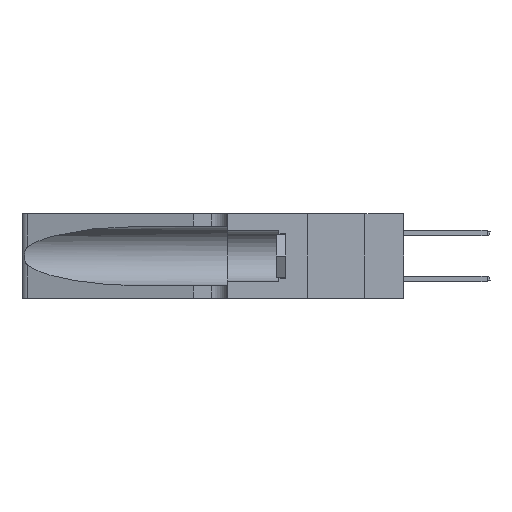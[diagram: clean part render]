
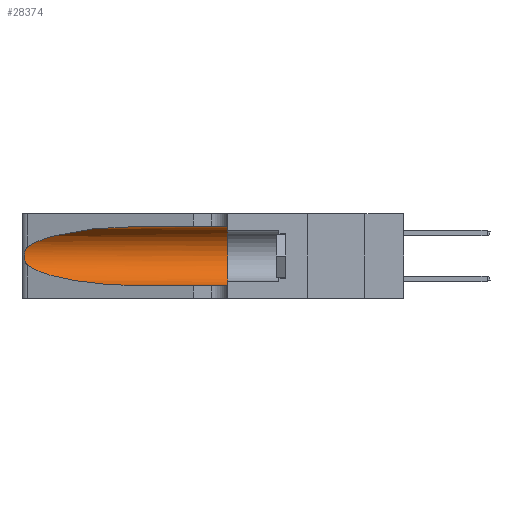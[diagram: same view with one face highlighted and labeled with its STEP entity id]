
A CAD part, left-side view. The second image highlights one B-rep face of the part: STEP entity #28374.
In plain terms, the highlighted cylindrical face has radius 3.308 mm (diameter 6.617 mm), a partial arc.
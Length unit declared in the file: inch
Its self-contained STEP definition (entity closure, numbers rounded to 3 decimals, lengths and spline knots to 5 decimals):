
#42 =( BOUNDED_CURVE ( )  B_SPLINE_CURVE ( 3, ( #224, #16903, #26453, #12285 ),
 .UNSPECIFIED., .F., .T. ) 
 B_SPLINE_CURVE_WITH_KNOTS ( ( 4, 4 ),
 ( 1.5708, 2.84003 ),
 .UNSPECIFIED. ) 
 CURVE ( )  GEOMETRIC_REPRESENTATION_ITEM ( )  RATIONAL_B_SPLINE_CURVE ( ( 1., 0.87, 0.87, 1. ) ) 
 REPRESENTATION_ITEM ( '' )  );
#224 = CARTESIAN_POINT ( 'NONE',  ( 0.1305, 0.72297, 0.31525 ) ) ;
#327 = VERTEX_POINT ( 'NONE', #13470 ) ;
#747 = CARTESIAN_POINT ( 'NONE',  ( 0.25856, 1.23593, 0.16098 ) ) ;
#1084 = EDGE_LOOP ( 'NONE', ( #18955, #22016, #24388, #9572, #19507, #29017 ) ) ;
#1754 = CARTESIAN_POINT ( 'NONE',  ( 0.2373, 1.15595, 0.08982 ) ) ;
#2404 = DIRECTION ( 'NONE',  ( 0., 0., -1. ) ) ;
#3135 = CARTESIAN_POINT ( 'NONE',  ( 0.25639, 1.23186, 0.15144 ) ) ;
#3586 = VERTEX_POINT ( 'NONE', #21520 ) ;
#4173 = CARTESIAN_POINT ( 'NONE',  ( 0.1305, 0.72297, 0.05475 ) ) ;
#5580 = CARTESIAN_POINT ( 'NONE',  ( 0.25487, 1.22718, 0.14631 ) ) ;
#7296 = DIRECTION ( 'NONE',  ( 0., -1., 0. ) ) ;
#7548 = B_SPLINE_CURVE_WITH_KNOTS ( 'NONE', 3,
 ( #19732, #22153, #7916, #24529, #10344, #26900, #12727, #29223, #15085, #747, #17449, #3135, #19835, #5580 ),
 .UNSPECIFIED., .F., .F.,
 ( 4, 2, 2, 2, 2, 2, 4 ),
 ( 0., 0.00027, 0.00053, 0.00107, 0.0016, 0.00187, 0.00214 ),
 .UNSPECIFIED. ) ;
#7802 =( BOUNDED_CURVE ( )  B_SPLINE_CURVE ( 3, ( #30227, #1754, #18464, #4173 ),
 .UNSPECIFIED., .F., .T. ) 
 B_SPLINE_CURVE_WITH_KNOTS ( ( 4, 4 ),
 ( 3.44316, 4.71239 ),
 .UNSPECIFIED. ) 
 CURVE ( )  GEOMETRIC_REPRESENTATION_ITEM ( )  RATIONAL_B_SPLINE_CURVE ( ( 1., 0.87, 0.87, 1. ) ) 
 REPRESENTATION_ITEM ( '' )  );
#7916 = CARTESIAN_POINT ( 'NONE',  ( 0.25639, 1.23184, 0.21858 ) ) ;
#8678 = DIRECTION ( 'NONE',  ( 0., -1., 0. ) ) ;
#9147 = CARTESIAN_POINT ( 'NONE',  ( 0.25487, 1.22718, 0.14631 ) ) ;
#9572 = ORIENTED_EDGE ( 'NONE', *, *, #24642, .T. ) ;
#9901 = VERTEX_POINT ( 'NONE', #20245 ) ;
#10058 = LINE ( 'NONE', #23966, #15610 ) ;
#10344 = CARTESIAN_POINT ( 'NONE',  ( 0.25854, 1.2359, 0.20912 ) ) ;
#10809 = VECTOR ( 'NONE', #8678, 39.37008 ) ;
#12167 = DIRECTION ( 'NONE',  ( 0., -1., 0. ) ) ;
#12285 = CARTESIAN_POINT ( 'NONE',  ( 0.25487, 1.22718, 0.22369 ) ) ;
#12727 = CARTESIAN_POINT ( 'NONE',  ( 0.26075, 1.23896, 0.19203 ) ) ;
#13013 = DIRECTION ( 'NONE',  ( 0., 1., 0. ) ) ;
#13470 = CARTESIAN_POINT ( 'NONE',  ( 0.1305, 0.35, 0.31525 ) ) ;
#13999 = AXIS2_PLACEMENT_3D ( 'NONE', #21553, #7296, #2404 ) ;
#15085 = CARTESIAN_POINT ( 'NONE',  ( 0.26017, 1.23833, 0.17102 ) ) ;
#15537 = CARTESIAN_POINT ( 'NONE',  ( 0.1305, 1.61858, 0.05475 ) ) ;
#15610 = VECTOR ( 'NONE', #12167, 39.37008 ) ;
#15941 = VERTEX_POINT ( 'NONE', #21848 ) ;
#16903 = CARTESIAN_POINT ( 'NONE',  ( 0.18966, 0.96281, 0.31525 ) ) ;
#17050 = LINE ( 'NONE', #15537, #10809 ) ;
#17211 = FACE_OUTER_BOUND ( 'NONE', #1084, .T. ) ;
#17449 = CARTESIAN_POINT ( 'NONE',  ( 0.25789, 1.23486, 0.15765 ) ) ;
#18464 = CARTESIAN_POINT ( 'NONE',  ( 0.18966, 0.96281, 0.05475 ) ) ;
#18955 = ORIENTED_EDGE ( 'NONE', *, *, #29144, .T. ) ;
#19507 = ORIENTED_EDGE ( 'NONE', *, *, #26562, .F. ) ;
#19732 = CARTESIAN_POINT ( 'NONE',  ( 0.25487, 1.22718, 0.22369 ) ) ;
#19835 = CARTESIAN_POINT ( 'NONE',  ( 0.25555, 1.22993, 0.14849 ) ) ;
#20245 = CARTESIAN_POINT ( 'NONE',  ( 0.1305, 0.72297, 0.05475 ) ) ;
#21520 = CARTESIAN_POINT ( 'NONE',  ( 0.1305, 0.35, 0.05475 ) ) ;
#21553 = CARTESIAN_POINT ( 'NONE',  ( 0.1305, 1.61858, 0.185 ) ) ;
#21848 = CARTESIAN_POINT ( 'NONE',  ( 0.25487, 1.22718, 0.22369 ) ) ;
#22016 = ORIENTED_EDGE ( 'NONE', *, *, #26650, .T. ) ;
#22153 = CARTESIAN_POINT ( 'NONE',  ( 0.25555, 1.22994, 0.2215 ) ) ;
#23414 = EDGE_CURVE ( 'NONE', #23438, #9901, #7802, .T. ) ;
#23438 = VERTEX_POINT ( 'NONE', #9147 ) ;
#23966 = CARTESIAN_POINT ( 'NONE',  ( 0.1305, 1.61858, 0.31525 ) ) ;
#24162 = AXIS2_PLACEMENT_3D ( 'NONE', #27156, #13013, #29489 ) ;
#24225 = EDGE_CURVE ( 'NONE', #27823, #327, #10058, .T. ) ;
#24388 = ORIENTED_EDGE ( 'NONE', *, *, #23414, .T. ) ;
#24529 = CARTESIAN_POINT ( 'NONE',  ( 0.25787, 1.23484, 0.2124 ) ) ;
#24642 = EDGE_CURVE ( 'NONE', #9901, #3586, #17050, .T. ) ;
#25367 = CIRCLE ( 'NONE', #24162, 0.13025 ) ;
#26121 = CARTESIAN_POINT ( 'NONE',  ( 0.1305, 0.72297, 0.31525 ) ) ;
#26453 = CARTESIAN_POINT ( 'NONE',  ( 0.2373, 1.15595, 0.28018 ) ) ;
#26562 = EDGE_CURVE ( 'NONE', #327, #3586, #25367, .T. ) ;
#26650 = EDGE_CURVE ( 'NONE', #15941, #23438, #7548, .T. ) ;
#26900 = CARTESIAN_POINT ( 'NONE',  ( 0.26018, 1.23835, 0.19895 ) ) ;
#27156 = CARTESIAN_POINT ( 'NONE',  ( 0.1305, 0.35, 0.185 ) ) ;
#27823 = VERTEX_POINT ( 'NONE', #26121 ) ;
#28374 = ADVANCED_FACE ( 'NONE', ( #17211 ), #29034, .F. ) ;
#29017 = ORIENTED_EDGE ( 'NONE', *, *, #24225, .F. ) ;
#29034 = CYLINDRICAL_SURFACE ( 'NONE', #13999, 0.13025 ) ;
#29144 = EDGE_CURVE ( 'NONE', #27823, #15941, #42, .T. ) ;
#29223 = CARTESIAN_POINT ( 'NONE',  ( 0.26075, 1.23896, 0.178 ) ) ;
#29489 = DIRECTION ( 'NONE',  ( 0., 0., 1. ) ) ;
#30227 = CARTESIAN_POINT ( 'NONE',  ( 0.25487, 1.22718, 0.14631 ) ) ;
